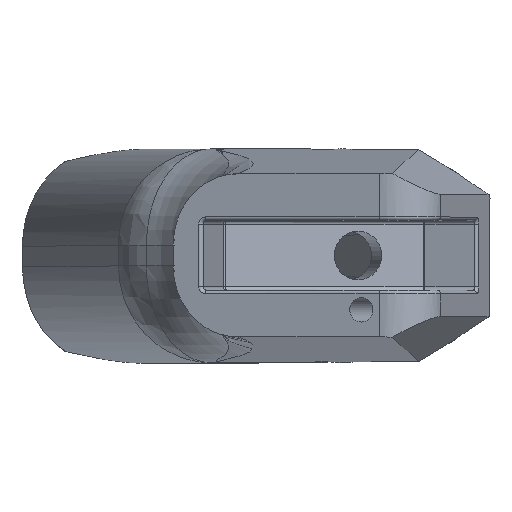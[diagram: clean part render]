
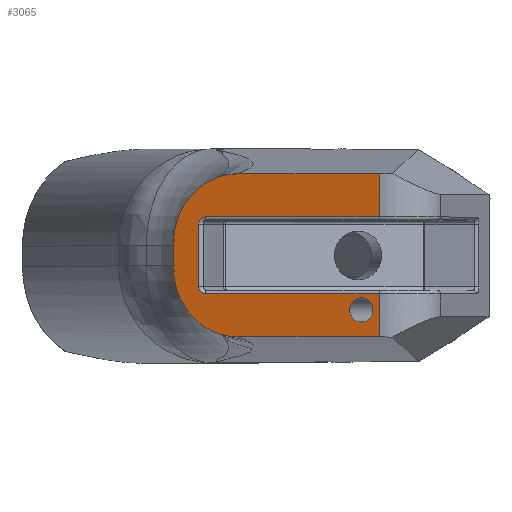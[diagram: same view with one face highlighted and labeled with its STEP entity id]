
A CAD part, top view. The second image highlights one B-rep face of the part: STEP entity #3065.
In plain terms, the highlighted planar face has unit normal (-0.292, 0, 0.956).
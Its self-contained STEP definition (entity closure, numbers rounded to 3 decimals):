
#52=FACE_BOUND('',#547,.T.);
#142=CIRCLE('',#3324,1.);
#143=CIRCLE('',#3325,1.);
#144=CIRCLE('',#3326,1.7);
#366=FACE_OUTER_BOUND('',#546,.T.);
#546=EDGE_LOOP('',(#2674,#2675,#2676,#2677,#2678,#2679,#2680,#2681,#2682,
#2683,#2684,#2685,#2686,#2687));
#547=EDGE_LOOP('',(#2688));
#703=LINE('',#5837,#890);
#706=LINE('',#5933,#893);
#730=LINE('',#6493,#917);
#746=LINE('',#6990,#933);
#747=LINE('',#6992,#934);
#748=LINE('',#6996,#935);
#749=LINE('',#7000,#936);
#750=LINE('',#7001,#937);
#890=VECTOR('',#3785,10.);
#893=VECTOR('',#3792,10.);
#917=VECTOR('',#3900,10.);
#933=VECTOR('',#3962,10.);
#934=VECTOR('',#3963,10.);
#935=VECTOR('',#3966,10.);
#936=VECTOR('',#3969,10.);
#937=VECTOR('',#3970,10.);
#1091=B_SPLINE_CURVE_WITH_KNOTS('',3,(#6518,#6519,#6520,#6521),
 .UNSPECIFIED.,.F.,.F.,(4,4),(3.986,4.024),
 .UNSPECIFIED.);
#1098=B_SPLINE_CURVE_WITH_KNOTS('',3,(#6904,#6905,#6906,#6907,#6908,#6909,
#6910,#6911,#6912,#6913,#6914,#6915),.UNSPECIFIED.,.F.,.F.,(4,2,2,2,2,4),
(0.,0.391,0.764,1.117,1.313,
1.493),.UNSPECIFIED.);
#1101=B_SPLINE_CURVE_WITH_KNOTS('',3,(#6975,#6976,#6977,#6978),
 .UNSPECIFIED.,.F.,.F.,(4,4),(4.024,4.062),
 .UNSPECIFIED.);
#1102=B_SPLINE_CURVE_WITH_KNOTS('',3,(#6979,#6980,#6981,#6982,#6983,#6984,
#6985,#6986,#6987,#6988),.UNSPECIFIED.,.F.,.F.,(4,2,2,2,4),(0.,0.358,
0.733,1.094,1.492),.UNSPECIFIED.);
#1354=VERTEX_POINT('',#5834);
#1355=VERTEX_POINT('',#5836);
#1358=VERTEX_POINT('',#5911);
#1359=VERTEX_POINT('',#5932);
#1390=VERTEX_POINT('',#6490);
#1391=VERTEX_POINT('',#6492);
#1392=VERTEX_POINT('',#6496);
#1415=VERTEX_POINT('',#6903);
#1416=VERTEX_POINT('',#6989);
#1417=VERTEX_POINT('',#6991);
#1418=VERTEX_POINT('',#6993);
#1419=VERTEX_POINT('',#6995);
#1420=VERTEX_POINT('',#6997);
#1421=VERTEX_POINT('',#6999);
#1422=VERTEX_POINT('',#7002);
#1737=EDGE_CURVE('',#1355,#1354,#703,.T.);
#1746=EDGE_CURVE('',#1359,#1358,#706,.T.);
#1811=EDGE_CURVE('',#1390,#1391,#730,.T.);
#1814=EDGE_CURVE('',#1392,#1390,#1091,.T.);
#1848=EDGE_CURVE('',#1415,#1358,#1098,.T.);
#1851=EDGE_CURVE('',#1391,#1415,#1101,.T.);
#1852=EDGE_CURVE('',#1355,#1392,#1102,.T.);
#1853=EDGE_CURVE('',#1416,#1354,#746,.T.);
#1854=EDGE_CURVE('',#1417,#1416,#747,.T.);
#1855=EDGE_CURVE('',#1418,#1417,#142,.T.);
#1856=EDGE_CURVE('',#1419,#1418,#748,.T.);
#1857=EDGE_CURVE('',#1420,#1419,#143,.T.);
#1858=EDGE_CURVE('',#1421,#1420,#749,.T.);
#1859=EDGE_CURVE('',#1421,#1359,#750,.T.);
#1860=EDGE_CURVE('',#1422,#1422,#144,.T.);
#2674=ORIENTED_EDGE('',*,*,#1848,.F.);
#2675=ORIENTED_EDGE('',*,*,#1851,.F.);
#2676=ORIENTED_EDGE('',*,*,#1811,.F.);
#2677=ORIENTED_EDGE('',*,*,#1814,.F.);
#2678=ORIENTED_EDGE('',*,*,#1852,.F.);
#2679=ORIENTED_EDGE('',*,*,#1737,.T.);
#2680=ORIENTED_EDGE('',*,*,#1853,.F.);
#2681=ORIENTED_EDGE('',*,*,#1854,.F.);
#2682=ORIENTED_EDGE('',*,*,#1855,.F.);
#2683=ORIENTED_EDGE('',*,*,#1856,.F.);
#2684=ORIENTED_EDGE('',*,*,#1857,.F.);
#2685=ORIENTED_EDGE('',*,*,#1858,.F.);
#2686=ORIENTED_EDGE('',*,*,#1859,.T.);
#2687=ORIENTED_EDGE('',*,*,#1746,.T.);
#2688=ORIENTED_EDGE('',*,*,#1860,.T.);
#2920=PLANE('',#3323);
#3065=ADVANCED_FACE('',(#366,#52),#2920,.F.);
#3323=AXIS2_PLACEMENT_3D('',#6974,#3960,#3961);
#3324=AXIS2_PLACEMENT_3D('',#6994,#3964,#3965);
#3325=AXIS2_PLACEMENT_3D('',#6998,#3967,#3968);
#3326=AXIS2_PLACEMENT_3D('',#7003,#3971,#3972);
#3785=DIRECTION('',(0.956,0.,0.292));
#3792=DIRECTION('',(-0.956,0.,-0.292));
#3900=DIRECTION('',(0.,1.,0.));
#3960=DIRECTION('center_axis',(0.292,0.,-0.956));
#3961=DIRECTION('ref_axis',(0.956,0.,0.292));
#3962=DIRECTION('',(0.,-1.,0.));
#3963=DIRECTION('',(0.956,0.,0.292));
#3964=DIRECTION('center_axis',(-0.292,0.,0.956));
#3965=DIRECTION('ref_axis',(-0.676,-0.707,-0.207));
#3966=DIRECTION('',(0.,-1.,0.));
#3967=DIRECTION('center_axis',(-0.292,0.,0.956));
#3968=DIRECTION('ref_axis',(-0.676,0.707,-0.207));
#3969=DIRECTION('',(-0.956,0.,-0.292));
#3970=DIRECTION('',(0.,1.,0.));
#3971=DIRECTION('center_axis',(0.292,0.,-0.956));
#3972=DIRECTION('ref_axis',(0.,1.,0.));
#5834=CARTESIAN_POINT('',(-2.498,-130.183,-121.464));
#5836=CARTESIAN_POINT('',(-22.213,-130.183,-127.491));
#5837=CARTESIAN_POINT('',(-11.242,-130.183,-124.137));
#5911=CARTESIAN_POINT('',(-22.213,-107.372,-127.491));
#5932=CARTESIAN_POINT('',(-2.498,-107.372,-121.463));
#5933=CARTESIAN_POINT('',(-11.242,-107.372,-124.137));
#6490=CARTESIAN_POINT('',(-31.262,-120.2,-130.258));
#6492=CARTESIAN_POINT('',(-31.262,-117.356,-130.258));
#6493=CARTESIAN_POINT('',(-31.262,-107.856,-130.258));
#6496=CARTESIAN_POINT('',(-31.257,-120.585,-130.256));
#6518=CARTESIAN_POINT('Ctrl Pts',(-31.257,-120.585,-130.256));
#6519=CARTESIAN_POINT('Ctrl Pts',(-31.261,-120.455,-130.257));
#6520=CARTESIAN_POINT('Ctrl Pts',(-31.262,-120.327,-130.258));
#6521=CARTESIAN_POINT('Ctrl Pts',(-31.262,-120.2,-130.258));
#6903=CARTESIAN_POINT('',(-31.257,-116.97,-130.256));
#6904=CARTESIAN_POINT('Ctrl Pts',(-31.257,-116.97,-130.256));
#6905=CARTESIAN_POINT('Ctrl Pts',(-31.22,-115.667,-130.245));
#6906=CARTESIAN_POINT('Ctrl Pts',(-30.943,-114.379,-130.16));
#6907=CARTESIAN_POINT('Ctrl Pts',(-29.968,-112.046,-129.862));
#6908=CARTESIAN_POINT('Ctrl Pts',(-29.296,-111.006,-129.657));
#6909=CARTESIAN_POINT('Ctrl Pts',(-27.661,-109.292,-129.157));
#6910=CARTESIAN_POINT('Ctrl Pts',(-26.728,-108.616,-128.871));
#6911=CARTESIAN_POINT('Ctrl Pts',(-25.128,-107.88,-128.382));
#6912=CARTESIAN_POINT('Ctrl Pts',(-24.534,-107.682,-128.201));
#6913=CARTESIAN_POINT('Ctrl Pts',(-23.361,-107.433,-127.842));
#6914=CARTESIAN_POINT('Ctrl Pts',(-22.788,-107.372,-127.667));
#6915=CARTESIAN_POINT('Ctrl Pts',(-22.213,-107.372,-127.491));
#6974=CARTESIAN_POINT('Origin',(-26.545,-107.856,-128.815));
#6975=CARTESIAN_POINT('Ctrl Pts',(-31.262,-117.356,-130.258));
#6976=CARTESIAN_POINT('Ctrl Pts',(-31.262,-117.229,-130.258));
#6977=CARTESIAN_POINT('Ctrl Pts',(-31.261,-117.1,-130.257));
#6978=CARTESIAN_POINT('Ctrl Pts',(-31.257,-116.97,-130.256));
#6979=CARTESIAN_POINT('Ctrl Pts',(-22.213,-130.183,-127.491));
#6980=CARTESIAN_POINT('Ctrl Pts',(-23.355,-130.183,-127.84));
#6981=CARTESIAN_POINT('Ctrl Pts',(-24.483,-129.944,-128.185));
#6982=CARTESIAN_POINT('Ctrl Pts',(-26.642,-129.003,-128.845));
#6983=CARTESIAN_POINT('Ctrl Pts',(-27.639,-128.293,-129.15));
#6984=CARTESIAN_POINT('Ctrl Pts',(-29.291,-126.548,-129.655));
#6985=CARTESIAN_POINT('Ctrl Pts',(-29.945,-125.541,-129.855));
#6986=CARTESIAN_POINT('Ctrl Pts',(-30.932,-123.227,-130.157));
#6987=CARTESIAN_POINT('Ctrl Pts',(-31.219,-121.914,-130.245));
#6988=CARTESIAN_POINT('Ctrl Pts',(-31.257,-120.585,-130.256));
#6989=CARTESIAN_POINT('',(-2.498,-124.14,-121.464));
#6990=CARTESIAN_POINT('',(-2.498,-129.7,-121.464));
#6991=CARTESIAN_POINT('',(-26.747,-124.14,-128.877));
#6992=CARTESIAN_POINT('',(-19.064,-124.14,-126.528));
#6993=CARTESIAN_POINT('',(-27.703,-123.14,-129.17));
#6994=CARTESIAN_POINT('Origin',(-26.747,-123.14,-128.877));
#6995=CARTESIAN_POINT('',(-27.703,-114.415,-129.17));
#6996=CARTESIAN_POINT('',(-27.703,-113.317,-129.17));
#6997=CARTESIAN_POINT('',(-26.747,-113.415,-128.877));
#6998=CARTESIAN_POINT('Origin',(-26.747,-114.415,-128.877));
#6999=CARTESIAN_POINT('',(-2.498,-113.415,-121.463));
#7000=CARTESIAN_POINT('',(-19.064,-113.415,-126.528));
#7001=CARTESIAN_POINT('',(-2.498,-107.856,-121.463));
#7002=CARTESIAN_POINT('',(-4.975,-128.1,-122.221));
#7003=CARTESIAN_POINT('Origin',(-4.975,-126.4,-122.221));
